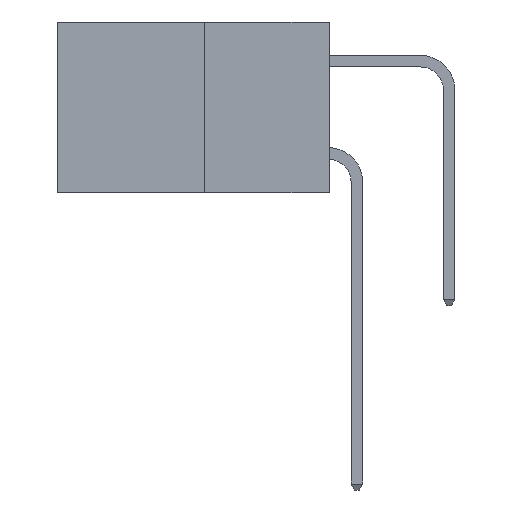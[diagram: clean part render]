
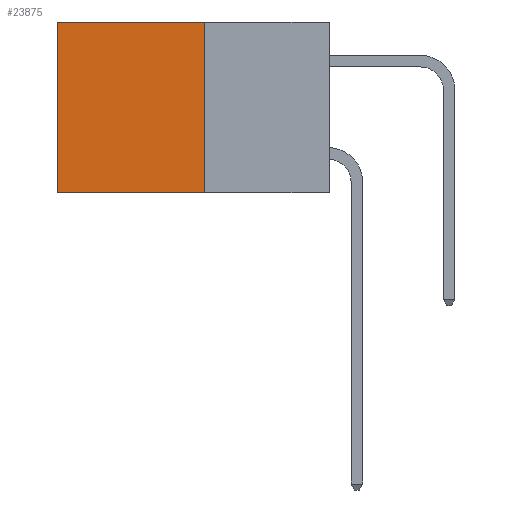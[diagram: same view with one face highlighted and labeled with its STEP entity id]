
A CAD part, left-side view. The second image highlights one B-rep face of the part: STEP entity #23875.
In plain terms, the highlighted planar face has unit normal (-1, 0, 0).
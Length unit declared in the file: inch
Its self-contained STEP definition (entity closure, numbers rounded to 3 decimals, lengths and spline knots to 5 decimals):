
#740 = CARTESIAN_POINT ( 'NONE',  ( 0.277, 0.27, -0.37 ) ) ;
#2670 = LINE ( 'NONE', #8855, #13117 ) ;
#2884 = CARTESIAN_POINT ( 'NONE',  ( 0.277, 0.27, -0.37 ) ) ;
#3126 = LINE ( 'NONE', #21331, #23830 ) ;
#3415 = VERTEX_POINT ( 'NONE', #2884 ) ;
#4713 = CARTESIAN_POINT ( 'NONE',  ( 0.277, 0.27, 0. ) ) ;
#6334 = FACE_OUTER_BOUND ( 'NONE', #14888, .T. ) ;
#6605 = DIRECTION ( 'NONE',  ( 0., 1., 0. ) ) ;
#6782 = CARTESIAN_POINT ( 'NONE',  ( 0.277, 0.27, -0.37 ) ) ;
#7046 = AXIS2_PLACEMENT_3D ( 'NONE', #20501, #8755, #22396 ) ;
#7666 = DIRECTION ( 'NONE',  ( 0., 1., 0. ) ) ;
#8118 = CARTESIAN_POINT ( 'NONE',  ( 0.277, 0.59, -0.37 ) ) ;
#8755 = DIRECTION ( 'NONE',  ( 1., 0., 0. ) ) ;
#8766 = DIRECTION ( 'NONE',  ( 0., 0., -1. ) ) ;
#8855 = CARTESIAN_POINT ( 'NONE',  ( 0.277, 0.59, -0.37 ) ) ;
#9614 = VERTEX_POINT ( 'NONE', #8118 ) ;
#10159 = EDGE_CURVE ( 'NONE', #22226, #11855, #3126, .T. ) ;
#10737 = ORIENTED_EDGE ( 'NONE', *, *, #22838, .T. ) ;
#11855 = VERTEX_POINT ( 'NONE', #16432 ) ;
#11991 = ORIENTED_EDGE ( 'NONE', *, *, #15089, .F. ) ;
#12191 = LINE ( 'NONE', #6782, #21877 ) ;
#12835 = LINE ( 'NONE', #740, #22519 ) ;
#12855 = DIRECTION ( 'NONE',  ( 0., 0., -1. ) ) ;
#13117 = VECTOR ( 'NONE', #12855, 39.37008 ) ;
#14888 = EDGE_LOOP ( 'NONE', ( #10737, #21080, #11991, #17151 ) ) ;
#15089 = EDGE_CURVE ( 'NONE', #22226, #3415, #12191, .T. ) ;
#16432 = CARTESIAN_POINT ( 'NONE',  ( 0.277, 0.59, 0. ) ) ;
#17151 = ORIENTED_EDGE ( 'NONE', *, *, #10159, .T. ) ;
#18439 = PLANE ( 'NONE',  #7046 ) ;
#20501 = CARTESIAN_POINT ( 'NONE',  ( 0.277, 0.27, -0.37 ) ) ;
#21080 = ORIENTED_EDGE ( 'NONE', *, *, #23802, .F. ) ;
#21331 = CARTESIAN_POINT ( 'NONE',  ( 0.277, 0.27, 0. ) ) ;
#21877 = VECTOR ( 'NONE', #8766, 39.37008 ) ;
#22226 = VERTEX_POINT ( 'NONE', #4713 ) ;
#22396 = DIRECTION ( 'NONE',  ( 0., 0., -1. ) ) ;
#22519 = VECTOR ( 'NONE', #6605, 39.37008 ) ;
#22838 = EDGE_CURVE ( 'NONE', #11855, #9614, #2670, .T. ) ;
#23802 = EDGE_CURVE ( 'NONE', #3415, #9614, #12835, .T. ) ;
#23830 = VECTOR ( 'NONE', #7666, 39.37008 ) ;
#23875 = ADVANCED_FACE ( 'NONE', ( #6334 ), #18439, .F. ) ;
